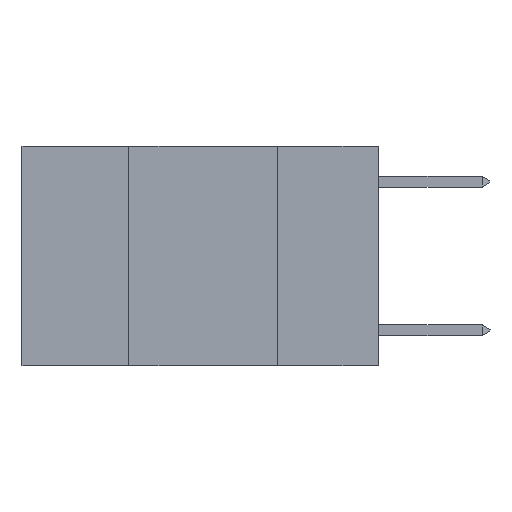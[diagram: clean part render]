
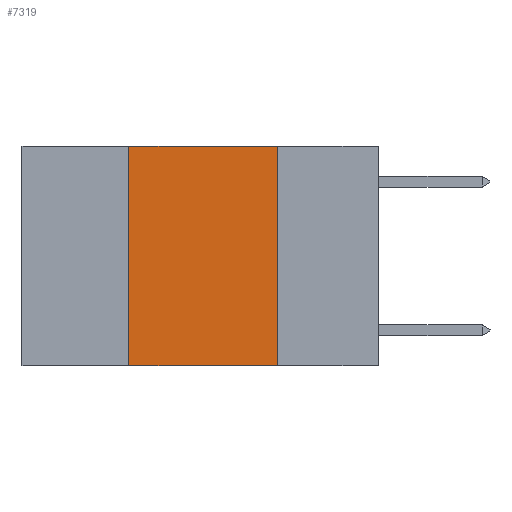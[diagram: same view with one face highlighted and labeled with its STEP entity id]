
A CAD part, left-side view. The second image highlights one B-rep face of the part: STEP entity #7319.
In plain terms, the highlighted planar face has unit normal (-1, 0, 0).
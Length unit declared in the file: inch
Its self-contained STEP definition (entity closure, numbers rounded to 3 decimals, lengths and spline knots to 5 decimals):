
#1480 = CARTESIAN_POINT ( 'NONE',  ( 0., 0.42, 0. ) ) ;
#3157 = EDGE_LOOP ( 'NONE', ( #9341, #17027, #20295, #22155 ) ) ;
#3524 = CARTESIAN_POINT ( 'NONE',  ( 0., 0.17, -0.37 ) ) ;
#3659 = FACE_OUTER_BOUND ( 'NONE', #3157, .T. ) ;
#4419 = VECTOR ( 'NONE', #10364, 39.37008 ) ;
#4554 = CARTESIAN_POINT ( 'NONE',  ( 0., 0.17, 0. ) ) ;
#6426 = EDGE_CURVE ( 'NONE', #18586, #12932, #11106, .T. ) ;
#6433 = VECTOR ( 'NONE', #7428, 39.37008 ) ;
#7319 = ADVANCED_FACE ( 'NONE', ( #3659 ), #21643, .F. ) ;
#7384 = CARTESIAN_POINT ( 'NONE',  ( 0., 0.6, 0. ) ) ;
#7428 = DIRECTION ( 'NONE',  ( 0., -1., 0. ) ) ;
#9341 = ORIENTED_EDGE ( 'NONE', *, *, #11065, .F. ) ;
#10088 = VERTEX_POINT ( 'NONE', #3524 ) ;
#10364 = DIRECTION ( 'NONE',  ( 0., 0., 1. ) ) ;
#10385 = EDGE_CURVE ( 'NONE', #16894, #10088, #22308, .T. ) ;
#10784 = CARTESIAN_POINT ( 'NONE',  ( 0., 0.42, 0. ) ) ;
#11065 = EDGE_CURVE ( 'NONE', #12932, #10088, #13487, .T. ) ;
#11106 = LINE ( 'NONE', #7384, #6433 ) ;
#11431 = AXIS2_PLACEMENT_3D ( 'NONE', #21828, #21571, #21533 ) ;
#12932 = VERTEX_POINT ( 'NONE', #14908 ) ;
#13487 = LINE ( 'NONE', #4554, #16984 ) ;
#14908 = CARTESIAN_POINT ( 'NONE',  ( 0., 0.17, 0. ) ) ;
#15079 = CARTESIAN_POINT ( 'NONE',  ( 0., 0.6, -0.37 ) ) ;
#16805 = DIRECTION ( 'NONE',  ( 0., -1., 0. ) ) ;
#16894 = VERTEX_POINT ( 'NONE', #21681 ) ;
#16984 = VECTOR ( 'NONE', #18565, 39.37008 ) ;
#17027 = ORIENTED_EDGE ( 'NONE', *, *, #6426, .F. ) ;
#17747 = EDGE_CURVE ( 'NONE', #16894, #18586, #18308, .T. ) ;
#18308 = LINE ( 'NONE', #1480, #4419 ) ;
#18565 = DIRECTION ( 'NONE',  ( 0., 0., -1. ) ) ;
#18586 = VERTEX_POINT ( 'NONE', #10784 ) ;
#20295 = ORIENTED_EDGE ( 'NONE', *, *, #17747, .F. ) ;
#21533 = DIRECTION ( 'NONE',  ( 0., 0., -1. ) ) ;
#21571 = DIRECTION ( 'NONE',  ( 1., 0., 0. ) ) ;
#21643 = PLANE ( 'NONE',  #11431 ) ;
#21681 = CARTESIAN_POINT ( 'NONE',  ( 0., 0.42, -0.37 ) ) ;
#21779 = VECTOR ( 'NONE', #16805, 39.37008 ) ;
#21828 = CARTESIAN_POINT ( 'NONE',  ( 0., 0.6, 0. ) ) ;
#22155 = ORIENTED_EDGE ( 'NONE', *, *, #10385, .T. ) ;
#22308 = LINE ( 'NONE', #15079, #21779 ) ;
